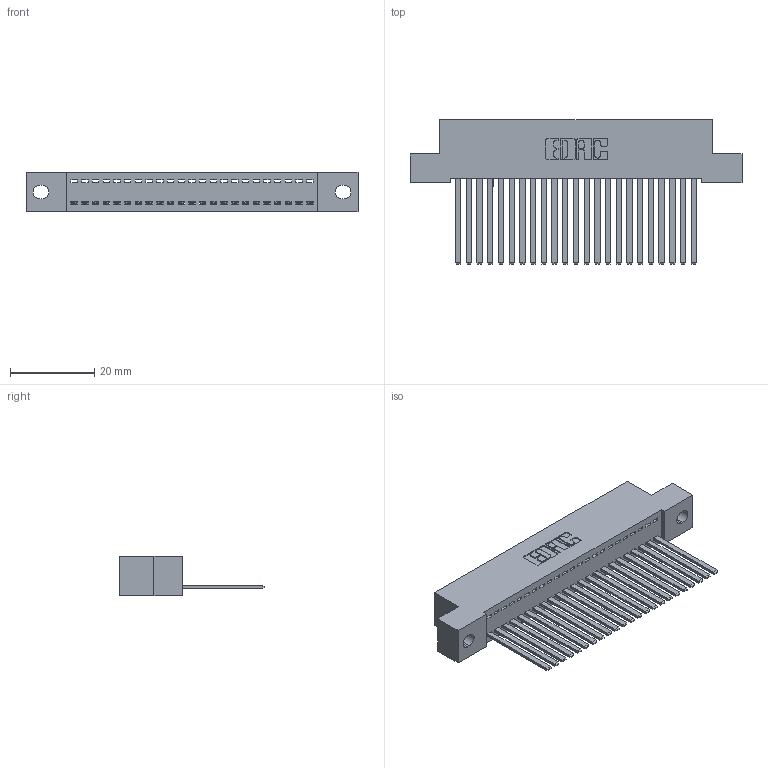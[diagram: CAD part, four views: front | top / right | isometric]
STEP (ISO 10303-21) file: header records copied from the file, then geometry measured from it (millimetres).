
FILE_DESCRIPTION (( 'STEP AP203' ), '1' );
FILE_NAME ('392-023-544-102.STEP', '2018-08-15T13:33:38', ( '' ), ( '' ), 'SwSTEP 2.0', 'SolidWorks 2016', '' );
FILE_SCHEMA (( 'CONFIG_CONTROL_DESIGN' ));
Length unit declared in the file: inch
Products named in the file (3): 342 Part_.128 Slot; 345-292-001_345-293-144; 392-023-544-102
Assembly tree (24 placements, depth 2):
  392-023-544-102
    342 Part_.128 Slot
    345-292-001_345-293-144  x23
Bounding box: 78.74 x 34.3 x 9.4 mm (x, y, z)
Volume: 7048.2 mm3; surface area: 10512.9 mm2
Topology: 24 solids, 24 shells, 1310 faces, 3945 edges, 2598 vertices
Faces by surface type: plane 944, cylinder 366
Entity records: 16337 total; most frequent: CARTESIAN_POINT 2827, ORIENTED_EDGE 2786, DIRECTION 2419, EDGE_CURVE 1393, VECTOR 1269, LINE 1269, VERTEX_POINT 926, AXIS2_PLACEMENT_3D 575
